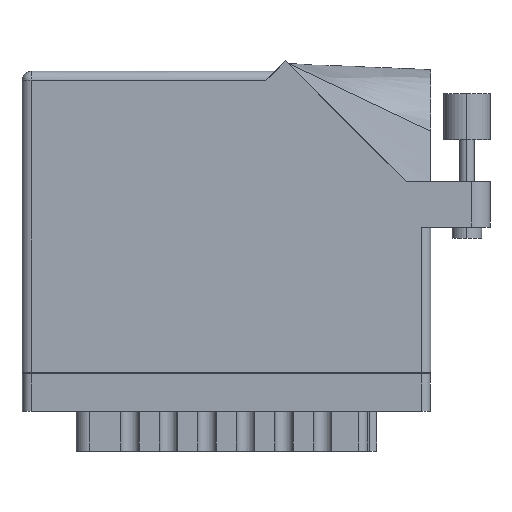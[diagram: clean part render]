
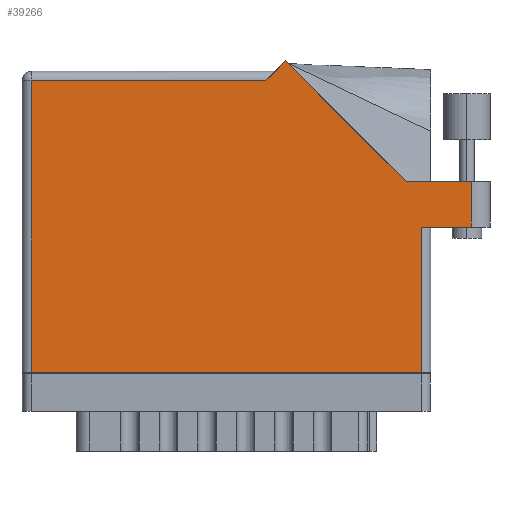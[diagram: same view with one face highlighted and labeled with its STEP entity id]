
A CAD part, front view. The second image highlights one B-rep face of the part: STEP entity #39266.
In plain terms, the highlighted face is planar.
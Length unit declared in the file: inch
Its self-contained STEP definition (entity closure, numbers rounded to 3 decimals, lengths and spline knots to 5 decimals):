
#303 = DIRECTION ( 'NONE',  ( -0.707, -0.707, 0. ) ) ;
#1210 = ORIENTED_EDGE ( 'NONE', *, *, #44268, .T. ) ;
#4403 = VECTOR ( 'NONE', #6978, 39.37008 ) ;
#5032 = EDGE_CURVE ( 'NONE', #23548, #30178, #33701, .T. ) ;
#6861 = VERTEX_POINT ( 'NONE', #82993 ) ;
#6978 = DIRECTION ( 'NONE',  ( -1., 0., 0. ) ) ;
#9723 = EDGE_CURVE ( 'NONE', #77976, #22531, #17920, .T. ) ;
#10023 = CARTESIAN_POINT ( 'NONE',  ( 3.03, 1.287, 0. ) ) ;
#10217 = VERTEX_POINT ( 'NONE', #50557 ) ;
#11546 = CARTESIAN_POINT ( 'NONE',  ( 2.58942, 1.287, 0. ) ) ;
#12434 = EDGE_CURVE ( 'NONE', #30178, #19796, #76027, .T. ) ;
#15769 = CARTESIAN_POINT ( 'NONE',  ( 3.03, 0.98, 0. ) ) ;
#16574 = ORIENTED_EDGE ( 'NONE', *, *, #5032, .T. ) ;
#17345 = DIRECTION ( 'NONE',  ( -0.707, 0.707, 0. ) ) ;
#17786 = CARTESIAN_POINT ( 'NONE',  ( 0., 0., 0. ) ) ;
#17920 = LINE ( 'NONE', #65513, #89540 ) ;
#19796 = VERTEX_POINT ( 'NONE', #53991 ) ;
#20915 = DIRECTION ( 'NONE',  ( 0., 1., 0. ) ) ;
#22531 = VERTEX_POINT ( 'NONE', #15769 ) ;
#23548 = VERTEX_POINT ( 'NONE', #82932 ) ;
#25176 = DIRECTION ( 'NONE',  ( -1., 0., 0. ) ) ;
#30178 = VERTEX_POINT ( 'NONE', #74081 ) ;
#33571 = EDGE_CURVE ( 'NONE', #42370, #23548, #71869, .T. ) ;
#33701 = LINE ( 'NONE', #63037, #46675 ) ;
#33736 = DIRECTION ( 'NONE',  ( 1., 0., 0. ) ) ;
#33895 = CARTESIAN_POINT ( 'NONE',  ( 3.03, 1.287, 0. ) ) ;
#33914 = VECTOR ( 'NONE', #20915, 39.37008 ) ;
#38370 = FACE_OUTER_BOUND ( 'NONE', #47929, .T. ) ;
#38937 = VECTOR ( 'NONE', #33736, 39.37008 ) ;
#39266 = ADVANCED_FACE ( 'NONE', ( #38370 ), #87393, .F. ) ;
#39373 = VECTOR ( 'NONE', #44069, 39.37008 ) ;
#40378 = ORIENTED_EDGE ( 'NONE', *, *, #12434, .T. ) ;
#42370 = VERTEX_POINT ( 'NONE', #11546 ) ;
#42495 = EDGE_CURVE ( 'NONE', #22531, #44884, #48122, .T. ) ;
#42660 = EDGE_CURVE ( 'NONE', #10217, #77976, #43698, .T. ) ;
#43698 = LINE ( 'NONE', #56604, #33914 ) ;
#44069 = DIRECTION ( 'NONE',  ( -1., 0., 0. ) ) ;
#44268 = EDGE_CURVE ( 'NONE', #19796, #6861, #48826, .T. ) ;
#44884 = VERTEX_POINT ( 'NONE', #10023 ) ;
#46675 = VECTOR ( 'NONE', #303, 39.37008 ) ;
#47929 = EDGE_LOOP ( 'NONE', ( #68826, #80598, #68981, #50395, #16574, #40378, #1210, #82297, #70189 ) ) ;
#48122 = LINE ( 'NONE', #33895, #52439 ) ;
#48826 = LINE ( 'NONE', #70744, #63941 ) ;
#50395 = ORIENTED_EDGE ( 'NONE', *, *, #33571, .T. ) ;
#50557 = CARTESIAN_POINT ( 'NONE',  ( 2.693, 0., 0. ) ) ;
#52306 = LINE ( 'NONE', #62813, #39373 ) ;
#52439 = VECTOR ( 'NONE', #61181, 39.37008 ) ;
#53991 = CARTESIAN_POINT ( 'NONE',  ( 0.062, 1.968, 0. ) ) ;
#55875 = EDGE_CURVE ( 'NONE', #44884, #42370, #52306, .T. ) ;
#56604 = CARTESIAN_POINT ( 'NONE',  ( 2.693, 0.98, 0. ) ) ;
#57380 = DIRECTION ( 'NONE',  ( 0., -1., 0. ) ) ;
#58221 = CARTESIAN_POINT ( 'NONE',  ( 2.58942, 1.287, 0. ) ) ;
#59641 = CARTESIAN_POINT ( 'NONE',  ( 2.693, 0.98, 0. ) ) ;
#59675 = CARTESIAN_POINT ( 'NONE',  ( 0., 2.03, 0. ) ) ;
#61181 = DIRECTION ( 'NONE',  ( 0., 1., 0. ) ) ;
#62813 = CARTESIAN_POINT ( 'NONE',  ( 3.155, 1.287, 0. ) ) ;
#63037 = CARTESIAN_POINT ( 'NONE',  ( 1.705, 2.03, 0. ) ) ;
#63941 = VECTOR ( 'NONE', #57380, 39.37008 ) ;
#65513 = CARTESIAN_POINT ( 'NONE',  ( 2.755, 0.98, 0. ) ) ;
#66682 = DIRECTION ( 'NONE',  ( 0., 0., -1. ) ) ;
#68826 = ORIENTED_EDGE ( 'NONE', *, *, #9723, .T. ) ;
#68981 = ORIENTED_EDGE ( 'NONE', *, *, #55875, .T. ) ;
#70189 = ORIENTED_EDGE ( 'NONE', *, *, #42660, .T. ) ;
#70744 = CARTESIAN_POINT ( 'NONE',  ( 0.062, 0., 0. ) ) ;
#71869 = LINE ( 'NONE', #58221, #89356 ) ;
#72775 = DIRECTION ( 'NONE',  ( 1., 0., 0. ) ) ;
#74081 = CARTESIAN_POINT ( 'NONE',  ( 1.643, 1.968, 0. ) ) ;
#76027 = LINE ( 'NONE', #90100, #4403 ) ;
#77976 = VERTEX_POINT ( 'NONE', #59641 ) ;
#80598 = ORIENTED_EDGE ( 'NONE', *, *, #42495, .T. ) ;
#82297 = ORIENTED_EDGE ( 'NONE', *, *, #84949, .T. ) ;
#82932 = CARTESIAN_POINT ( 'NONE',  ( 1.77571, 2.10071, 0. ) ) ;
#82993 = CARTESIAN_POINT ( 'NONE',  ( 0.062, 0., 0. ) ) ;
#83826 = AXIS2_PLACEMENT_3D ( 'NONE', #59675, #66682, #25176 ) ;
#84620 = LINE ( 'NONE', #17786, #38937 ) ;
#84949 = EDGE_CURVE ( 'NONE', #6861, #10217, #84620, .T. ) ;
#87393 = PLANE ( 'NONE',  #83826 ) ;
#89356 = VECTOR ( 'NONE', #17345, 39.37008 ) ;
#89540 = VECTOR ( 'NONE', #72775, 39.37008 ) ;
#90100 = CARTESIAN_POINT ( 'NONE',  ( 0., 1.968, 0. ) ) ;
